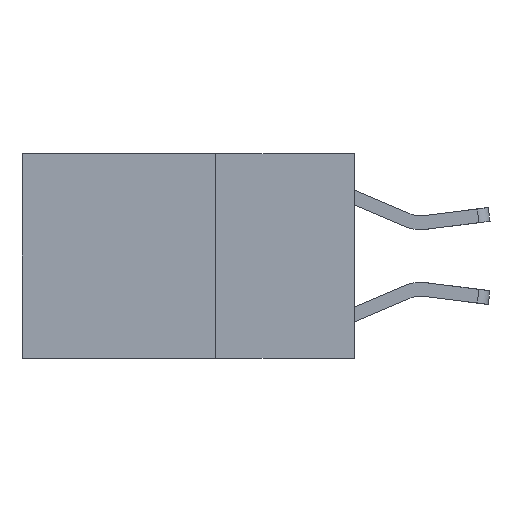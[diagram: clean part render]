
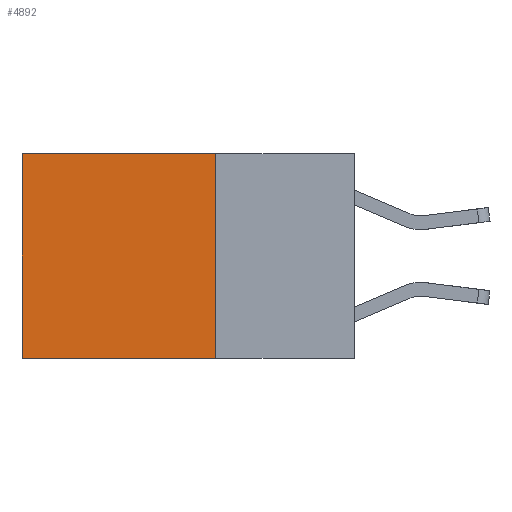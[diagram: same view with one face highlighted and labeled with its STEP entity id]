
A CAD part, left-side view. The second image highlights one B-rep face of the part: STEP entity #4892.
In plain terms, the highlighted planar face has unit normal (-1, 0, 0).
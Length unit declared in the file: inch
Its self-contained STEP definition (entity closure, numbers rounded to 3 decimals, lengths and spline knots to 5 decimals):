
#194 = VERTEX_POINT ( 'NONE', #2943 ) ;
#1020 = VECTOR ( 'NONE', #2941, 39.37008 ) ;
#1189 = EDGE_CURVE ( 'NONE', #7946, #194, #3234, .T. ) ;
#1294 = CARTESIAN_POINT ( 'NONE',  ( 0.2625, 0.25, 0. ) ) ;
#2096 = ORIENTED_EDGE ( 'NONE', *, *, #8599, .F. ) ;
#2098 = EDGE_LOOP ( 'NONE', ( #5120, #3369, #2096, #8246 ) ) ;
#2442 = LINE ( 'NONE', #3672, #6117 ) ;
#2535 = AXIS2_PLACEMENT_3D ( 'NONE', #3450, #7123, #2717 ) ;
#2651 = VECTOR ( 'NONE', #2701, 39.37008 ) ;
#2701 = DIRECTION ( 'NONE',  ( 0., 0., -1. ) ) ;
#2717 = DIRECTION ( 'NONE',  ( 0., 0., -1. ) ) ;
#2718 = FACE_OUTER_BOUND ( 'NONE', #2098, .T. ) ;
#2941 = DIRECTION ( 'NONE',  ( 0., 0., -1. ) ) ;
#2943 = CARTESIAN_POINT ( 'NONE',  ( 0.2625, 0.6, 0. ) ) ;
#3198 = LINE ( 'NONE', #6597, #1020 ) ;
#3234 = LINE ( 'NONE', #7275, #6908 ) ;
#3369 = ORIENTED_EDGE ( 'NONE', *, *, #8118, .F. ) ;
#3450 = CARTESIAN_POINT ( 'NONE',  ( 0.2625, 0.25, 0. ) ) ;
#3464 = CARTESIAN_POINT ( 'NONE',  ( 0.2625, 0.25, 0. ) ) ;
#3672 = CARTESIAN_POINT ( 'NONE',  ( 0.2625, 0.25, -0.37 ) ) ;
#3878 = EDGE_CURVE ( 'NONE', #194, #5381, #3198, .T. ) ;
#4871 = CARTESIAN_POINT ( 'NONE',  ( 0.2625, 0.6, -0.37 ) ) ;
#4892 = ADVANCED_FACE ( 'NONE', ( #2718 ), #6385, .F. ) ;
#5120 = ORIENTED_EDGE ( 'NONE', *, *, #3878, .T. ) ;
#5157 = DIRECTION ( 'NONE',  ( 0., 1., 0. ) ) ;
#5381 = VERTEX_POINT ( 'NONE', #4871 ) ;
#6117 = VECTOR ( 'NONE', #5157, 39.37008 ) ;
#6385 = PLANE ( 'NONE',  #2535 ) ;
#6597 = CARTESIAN_POINT ( 'NONE',  ( 0.2625, 0.6, 0. ) ) ;
#6908 = VECTOR ( 'NONE', #7402, 39.37008 ) ;
#7123 = DIRECTION ( 'NONE',  ( 1., 0., 0. ) ) ;
#7146 = CARTESIAN_POINT ( 'NONE',  ( 0.2625, 0.25, -0.37 ) ) ;
#7250 = VERTEX_POINT ( 'NONE', #7146 ) ;
#7275 = CARTESIAN_POINT ( 'NONE',  ( 0.2625, 0.25, 0. ) ) ;
#7402 = DIRECTION ( 'NONE',  ( 0., 1., 0. ) ) ;
#7946 = VERTEX_POINT ( 'NONE', #1294 ) ;
#8118 = EDGE_CURVE ( 'NONE', #7250, #5381, #2442, .T. ) ;
#8246 = ORIENTED_EDGE ( 'NONE', *, *, #1189, .T. ) ;
#8445 = LINE ( 'NONE', #3464, #2651 ) ;
#8599 = EDGE_CURVE ( 'NONE', #7946, #7250, #8445, .T. ) ;
